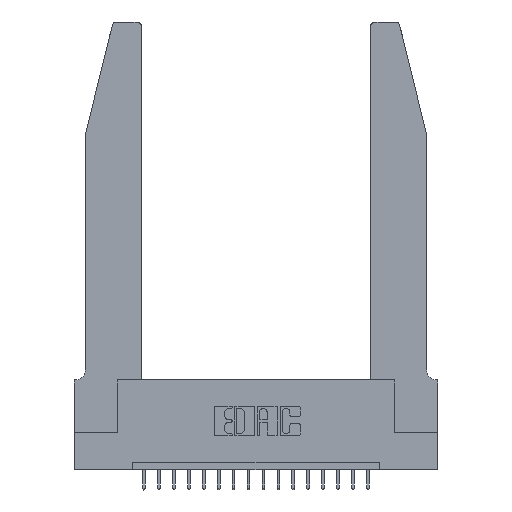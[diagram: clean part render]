
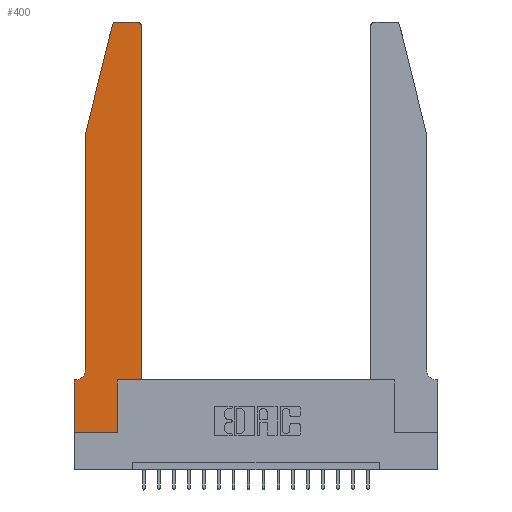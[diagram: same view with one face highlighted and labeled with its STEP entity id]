
A CAD part, top view. The second image highlights one B-rep face of the part: STEP entity #400.
In plain terms, the highlighted planar face has unit normal (0, 0, 1).
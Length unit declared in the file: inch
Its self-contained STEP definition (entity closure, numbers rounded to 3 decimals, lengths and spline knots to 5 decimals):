
#313 = AXIS2_PLACEMENT_3D ( 'NONE', #7592, #2641, #15400 ) ;
#354 = ORIENTED_EDGE ( 'NONE', *, *, #8909, .T. ) ;
#400 = ADVANCED_FACE ( 'NONE', ( #4415 ), #12190, .T. ) ;
#1463 = ORIENTED_EDGE ( 'NONE', *, *, #5634, .T. ) ;
#1600 = VERTEX_POINT ( 'NONE', #16404 ) ;
#2106 = EDGE_CURVE ( 'NONE', #1600, #13404, #10482, .T. ) ;
#2144 = DIRECTION ( 'NONE',  ( 1., 0., 0. ) ) ;
#2195 = EDGE_CURVE ( 'NONE', #12753, #8415, #15248, .T. ) ;
#2367 = ORIENTED_EDGE ( 'NONE', *, *, #2195, .T. ) ;
#2528 = ORIENTED_EDGE ( 'NONE', *, *, #20037, .T. ) ;
#2537 = ORIENTED_EDGE ( 'NONE', *, *, #8628, .T. ) ;
#2641 = DIRECTION ( 'NONE',  ( 0., 0., 1. ) ) ;
#3155 = EDGE_LOOP ( 'NONE', ( #10705, #1463, #2528, #2537, #2367, #17810, #11521, #19380, #354, #19342, #7688, #5316 ) ) ;
#3587 = DIRECTION ( 'NONE',  ( 0., 0., 1. ) ) ;
#3997 = CARTESIAN_POINT ( 'NONE',  ( 0.0755, 0.42, 0.37 ) ) ;
#4002 = CARTESIAN_POINT ( 'NONE',  ( 0.4205, 2.75, 0.37 ) ) ;
#4170 = VECTOR ( 'NONE', #12458, 39.37008 ) ;
#4415 = FACE_OUTER_BOUND ( 'NONE', #3155, .T. ) ;
#4473 = CARTESIAN_POINT ( 'NONE',  ( 0.0055, 0.42, 0.37 ) ) ;
#4721 = AXIS2_PLACEMENT_3D ( 'NONE', #5239, #17873, #2144 ) ;
#4960 = LINE ( 'NONE', #12932, #14918 ) ;
#5239 = CARTESIAN_POINT ( 'NONE',  ( 0.284, 2.72, 0.37 ) ) ;
#5316 = ORIENTED_EDGE ( 'NONE', *, *, #6102, .T. ) ;
#5319 = CARTESIAN_POINT ( 'NONE',  ( 0., 0., 0.37 ) ) ;
#5382 = CARTESIAN_POINT ( 'NONE',  ( 0., 0., 0.37 ) ) ;
#5634 = EDGE_CURVE ( 'NONE', #13805, #12528, #7019, .T. ) ;
#5787 = CARTESIAN_POINT ( 'NONE',  ( 0.4505, 0.35, 0.37 ) ) ;
#5913 = DIRECTION ( 'NONE',  ( -1., 0., 0. ) ) ;
#6102 = EDGE_CURVE ( 'NONE', #13404, #17837, #18920, .T. ) ;
#6220 = VERTEX_POINT ( 'NONE', #13742 ) ;
#6339 = VERTEX_POINT ( 'NONE', #11157 ) ;
#6472 = EDGE_CURVE ( 'NONE', #17515, #8642, #19466, .T. ) ;
#7012 = DIRECTION ( 'NONE',  ( 0., -1., 0. ) ) ;
#7019 = CIRCLE ( 'NONE', #4721, 0.03 ) ;
#7592 = CARTESIAN_POINT ( 'NONE',  ( 0., 0.35, 0.37 ) ) ;
#7688 = ORIENTED_EDGE ( 'NONE', *, *, #2106, .T. ) ;
#7909 = CARTESIAN_POINT ( 'NONE',  ( 0.2865, 0., 0.37 ) ) ;
#7946 = EDGE_CURVE ( 'NONE', #17837, #13805, #8143, .T. ) ;
#8143 = LINE ( 'NONE', #14498, #16685 ) ;
#8296 = CARTESIAN_POINT ( 'NONE',  ( 0.284, 2.75, 0.37 ) ) ;
#8415 = VERTEX_POINT ( 'NONE', #9251 ) ;
#8597 = VECTOR ( 'NONE', #13483, 39.37008 ) ;
#8628 = EDGE_CURVE ( 'NONE', #6220, #12753, #10835, .T. ) ;
#8642 = VERTEX_POINT ( 'NONE', #7909 ) ;
#8909 = EDGE_CURVE ( 'NONE', #8642, #6339, #10798, .T. ) ;
#9251 = CARTESIAN_POINT ( 'NONE',  ( 0.0055, 0.35, 0.37 ) ) ;
#10028 = CARTESIAN_POINT ( 'NONE',  ( 0.4205, 2.72, 0.37 ) ) ;
#10482 = LINE ( 'NONE', #18332, #8597 ) ;
#10705 = ORIENTED_EDGE ( 'NONE', *, *, #7946, .T. ) ;
#10797 = DIRECTION ( 'NONE',  ( -0.239, -0.971, 0. ) ) ;
#10798 = LINE ( 'NONE', #12252, #4170 ) ;
#10835 = LINE ( 'NONE', #17053, #14110 ) ;
#10946 = DIRECTION ( 'NONE',  ( 0., -1., 0. ) ) ;
#11157 = CARTESIAN_POINT ( 'NONE',  ( 0.2865, 0.35, 0.37 ) ) ;
#11521 = ORIENTED_EDGE ( 'NONE', *, *, #18937, .T. ) ;
#11693 = DIRECTION ( 'NONE',  ( 1., 0., 0. ) ) ;
#11875 = CARTESIAN_POINT ( 'NONE',  ( 0.4505, 2.72, 0.37 ) ) ;
#11922 = VECTOR ( 'NONE', #7012, 39.37008 ) ;
#12044 = LINE ( 'NONE', #13788, #18751 ) ;
#12190 = PLANE ( 'NONE',  #313 ) ;
#12252 = CARTESIAN_POINT ( 'NONE',  ( 0.2865, 0.35, 0.37 ) ) ;
#12458 = DIRECTION ( 'NONE',  ( 0., 1., 0. ) ) ;
#12528 = VERTEX_POINT ( 'NONE', #19395 ) ;
#12753 = VERTEX_POINT ( 'NONE', #3997 ) ;
#12830 = DIRECTION ( 'NONE',  ( 0., 0., -1. ) ) ;
#12932 = CARTESIAN_POINT ( 'NONE',  ( 0.0755, 2., 0.37 ) ) ;
#13362 = LINE ( 'NONE', #5787, #13847 ) ;
#13404 = VERTEX_POINT ( 'NONE', #11875 ) ;
#13483 = DIRECTION ( 'NONE',  ( 0., 1., 0. ) ) ;
#13742 = CARTESIAN_POINT ( 'NONE',  ( 0.0755, 2., 0.37 ) ) ;
#13788 = CARTESIAN_POINT ( 'NONE',  ( 0.0755, 0.35, 0.37 ) ) ;
#13805 = VERTEX_POINT ( 'NONE', #8296 ) ;
#13847 = VECTOR ( 'NONE', #19629, 39.37008 ) ;
#13924 = AXIS2_PLACEMENT_3D ( 'NONE', #4473, #12830, #15570 ) ;
#14110 = VECTOR ( 'NONE', #10946, 39.37008 ) ;
#14498 = CARTESIAN_POINT ( 'NONE',  ( 0.2605, 2.75, 0.37 ) ) ;
#14918 = VECTOR ( 'NONE', #10797, 39.37008 ) ;
#15248 = CIRCLE ( 'NONE', #13924, 0.07 ) ;
#15400 = DIRECTION ( 'NONE',  ( 1., 0., 0. ) ) ;
#15454 = CARTESIAN_POINT ( 'NONE',  ( 0., 0.35, 0.37 ) ) ;
#15570 = DIRECTION ( 'NONE',  ( -1., 0., 0. ) ) ;
#15764 = EDGE_CURVE ( 'NONE', #6339, #1600, #13362, .T. ) ;
#16216 = DIRECTION ( 'NONE',  ( 1., 0., 0. ) ) ;
#16404 = CARTESIAN_POINT ( 'NONE',  ( 0.4505, 0.35, 0.37 ) ) ;
#16656 = LINE ( 'NONE', #17884, #11922 ) ;
#16685 = VECTOR ( 'NONE', #17686, 39.37008 ) ;
#17053 = CARTESIAN_POINT ( 'NONE',  ( 0.0755, 2., 0.37 ) ) ;
#17191 = EDGE_CURVE ( 'NONE', #8415, #18260, #12044, .T. ) ;
#17515 = VERTEX_POINT ( 'NONE', #5382 ) ;
#17686 = DIRECTION ( 'NONE',  ( -1., 0., 0. ) ) ;
#17810 = ORIENTED_EDGE ( 'NONE', *, *, #17191, .T. ) ;
#17837 = VERTEX_POINT ( 'NONE', #4002 ) ;
#17873 = DIRECTION ( 'NONE',  ( 0., 0., 1. ) ) ;
#17884 = CARTESIAN_POINT ( 'NONE',  ( 0., 0., 0.37 ) ) ;
#17933 = AXIS2_PLACEMENT_3D ( 'NONE', #10028, #3587, #11693 ) ;
#18260 = VERTEX_POINT ( 'NONE', #15454 ) ;
#18332 = CARTESIAN_POINT ( 'NONE',  ( 0.4505, 0.35, 0.37 ) ) ;
#18751 = VECTOR ( 'NONE', #5913, 39.37008 ) ;
#18920 = CIRCLE ( 'NONE', #17933, 0.03 ) ;
#18937 = EDGE_CURVE ( 'NONE', #18260, #17515, #16656, .T. ) ;
#19342 = ORIENTED_EDGE ( 'NONE', *, *, #15764, .T. ) ;
#19380 = ORIENTED_EDGE ( 'NONE', *, *, #6472, .T. ) ;
#19395 = CARTESIAN_POINT ( 'NONE',  ( 0.25487, 2.72718, 0.37 ) ) ;
#19466 = LINE ( 'NONE', #5319, #19884 ) ;
#19629 = DIRECTION ( 'NONE',  ( 1., 0., 0. ) ) ;
#19884 = VECTOR ( 'NONE', #16216, 39.37008 ) ;
#20037 = EDGE_CURVE ( 'NONE', #12528, #6220, #4960, .T. ) ;
